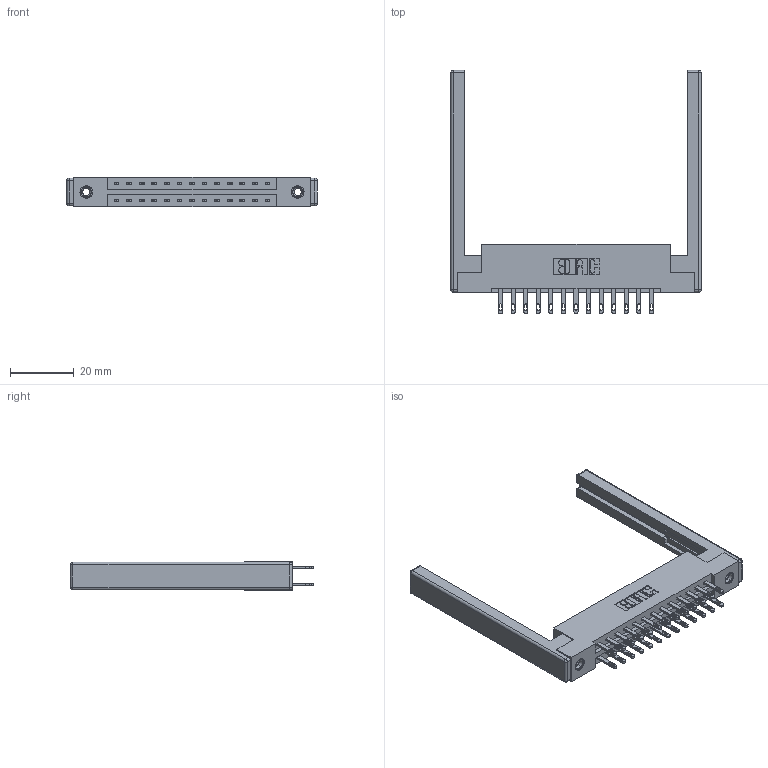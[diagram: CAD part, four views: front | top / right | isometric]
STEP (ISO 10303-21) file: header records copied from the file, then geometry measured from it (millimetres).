
FILE_DESCRIPTION (( 'STEP AP203' ), '1' );
FILE_NAME ('337-026-500-268.STEP', '2019-10-08T15:54:46', ( '' ), ( '' ), 'SwSTEP 2.0', 'SolidWorks 2016', '' );
FILE_SCHEMA (( 'CONFIG_CONTROL_DESIGN' ));
Length unit declared in the file: inch
Products named in the file (5): 345-292-001_345-293-100; 337 Part_Flush Mounting Lugs - 0.156 Dia-TI; 337-026-500-268; 307-220-068; 345-250-001_345-250-001-102
Assembly tree (31 placements, depth 2):
  337-026-500-268
    337 Part_Flush Mounting Lugs - 0.156 Dia-TI
    345-292-001_345-293-100  x26
    345-250-001_345-250-001-102  x2
    307-220-068  x2
Bounding box: 78.94 x 76.59 x 9.4 mm (x, y, z)
Volume: 12397.9 mm3; surface area: 13100 mm2
Topology: 31 solids, 31 shells, 1568 faces, 4679 edges, 3098 vertices
Faces by surface type: plane 990, cylinder 554, cone 12, sphere 8, torus 4
Entity records: 16520 total; most frequent: CARTESIAN_POINT 2771, ORIENTED_EDGE 2696, DIRECTION 2482, EDGE_CURVE 1348, VECTOR 1166, LINE 1166, VERTEX_POINT 890, AXIS2_PLACEMENT_3D 658
